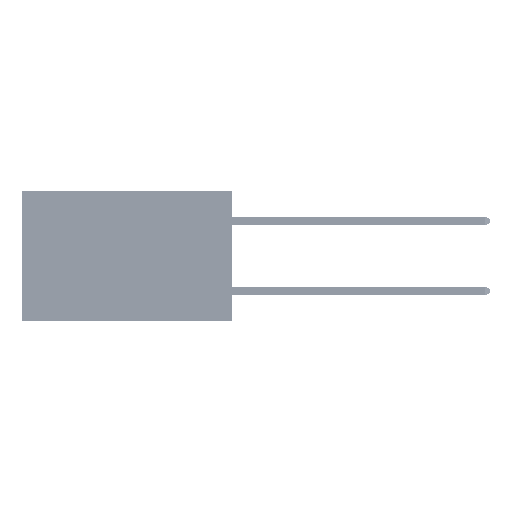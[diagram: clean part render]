
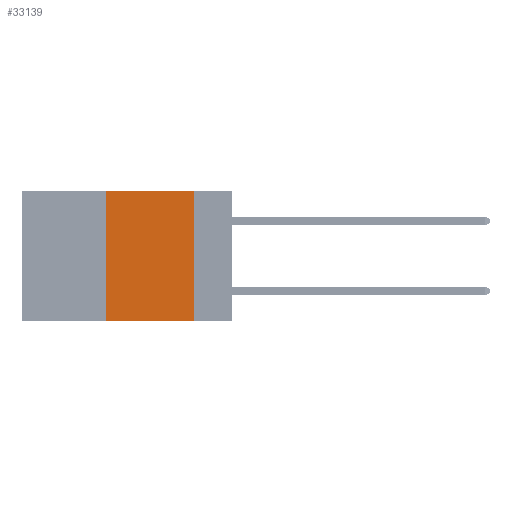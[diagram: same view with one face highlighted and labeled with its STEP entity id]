
A CAD part, left-side view. The second image highlights one B-rep face of the part: STEP entity #33139.
In plain terms, the highlighted planar face has unit normal (-1, 0, 0).
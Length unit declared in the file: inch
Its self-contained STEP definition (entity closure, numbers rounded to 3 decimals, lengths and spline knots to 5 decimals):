
#937 = DIRECTION ( 'NONE',  ( 0., -1., 0. ) ) ;
#1833 = CARTESIAN_POINT ( 'NONE',  ( 0., 0.36, 0. ) ) ;
#2631 = PLANE ( 'NONE',  #7777 ) ;
#7777 = AXIS2_PLACEMENT_3D ( 'NONE', #40958, #25095, #49022 ) ;
#8702 = VECTOR ( 'NONE', #42518, 39.37008 ) ;
#9975 = ORIENTED_EDGE ( 'NONE', *, *, #26682, .F. ) ;
#14563 = ORIENTED_EDGE ( 'NONE', *, *, #35217, .F. ) ;
#16468 = CARTESIAN_POINT ( 'NONE',  ( 0., 0.11, -0.37 ) ) ;
#19448 = EDGE_CURVE ( 'NONE', #48018, #24193, #20109, .T. ) ;
#19830 = CARTESIAN_POINT ( 'NONE',  ( 0., 0.36, 0. ) ) ;
#20109 = LINE ( 'NONE', #35484, #36464 ) ;
#20965 = DIRECTION ( 'NONE',  ( 0., -1., 0. ) ) ;
#20997 = DIRECTION ( 'NONE',  ( 0., 0., 1. ) ) ;
#21356 = VERTEX_POINT ( 'NONE', #22482 ) ;
#22054 = EDGE_LOOP ( 'NONE', ( #14563, #33680, #9975, #37942 ) ) ;
#22482 = CARTESIAN_POINT ( 'NONE',  ( 0., 0.11, 0. ) ) ;
#24193 = VERTEX_POINT ( 'NONE', #16468 ) ;
#24742 = LINE ( 'NONE', #40120, #41965 ) ;
#25095 = DIRECTION ( 'NONE',  ( 1., 0., 0. ) ) ;
#26682 = EDGE_CURVE ( 'NONE', #48018, #34074, #44185, .T. ) ;
#31747 = CARTESIAN_POINT ( 'NONE',  ( 0., 0.36, -0.37 ) ) ;
#33139 = ADVANCED_FACE ( 'NONE', ( #36931 ), #2631, .F. ) ;
#33680 = ORIENTED_EDGE ( 'NONE', *, *, #47814, .F. ) ;
#34074 = VERTEX_POINT ( 'NONE', #19830 ) ;
#35217 = EDGE_CURVE ( 'NONE', #21356, #24193, #49344, .T. ) ;
#35484 = CARTESIAN_POINT ( 'NONE',  ( 0., 0.6, -0.37 ) ) ;
#36464 = VECTOR ( 'NONE', #937, 39.37008 ) ;
#36931 = FACE_OUTER_BOUND ( 'NONE', #22054, .T. ) ;
#37942 = ORIENTED_EDGE ( 'NONE', *, *, #19448, .T. ) ;
#38253 = CARTESIAN_POINT ( 'NONE',  ( 0., 0.11, 0. ) ) ;
#40120 = CARTESIAN_POINT ( 'NONE',  ( 0., 0.6, 0. ) ) ;
#40958 = CARTESIAN_POINT ( 'NONE',  ( 0., 0.6, 0. ) ) ;
#41965 = VECTOR ( 'NONE', #20965, 39.37008 ) ;
#42518 = DIRECTION ( 'NONE',  ( 0., 0., -1. ) ) ;
#44185 = LINE ( 'NONE', #1833, #48517 ) ;
#47814 = EDGE_CURVE ( 'NONE', #34074, #21356, #24742, .T. ) ;
#48018 = VERTEX_POINT ( 'NONE', #31747 ) ;
#48517 = VECTOR ( 'NONE', #20997, 39.37008 ) ;
#49022 = DIRECTION ( 'NONE',  ( 0., 0., -1. ) ) ;
#49344 = LINE ( 'NONE', #38253, #8702 ) ;
